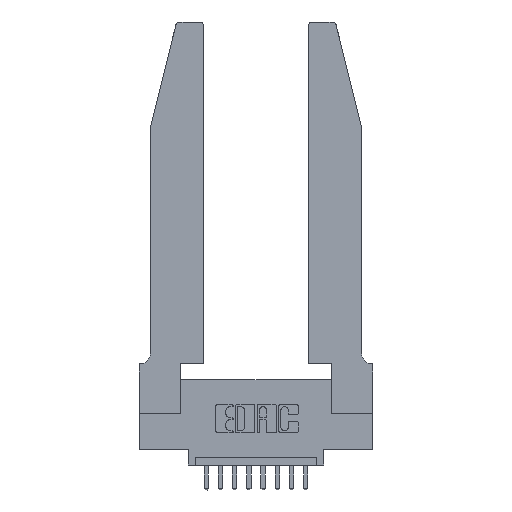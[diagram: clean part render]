
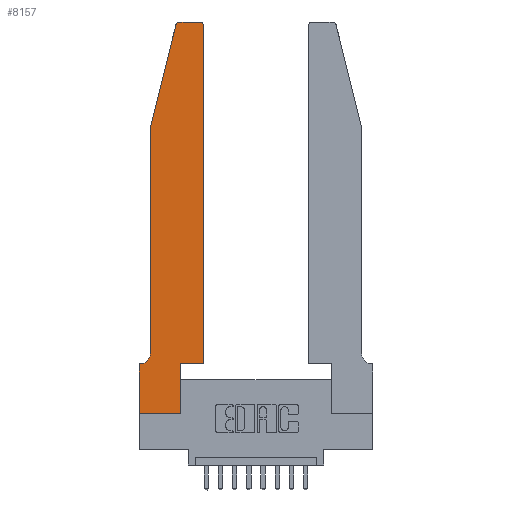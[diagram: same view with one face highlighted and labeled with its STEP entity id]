
A CAD part, top view. The second image highlights one B-rep face of the part: STEP entity #8157.
In plain terms, the highlighted planar face has unit normal (0, 0, 1).
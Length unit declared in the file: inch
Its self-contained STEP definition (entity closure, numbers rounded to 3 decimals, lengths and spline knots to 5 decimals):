
#4 = VECTOR ( 'NONE', #285, 39.37008 ) ;
#128 = EDGE_CURVE ( 'NONE', #5290, #318, #14136, .T. ) ;
#135 = CIRCLE ( 'NONE', #1114, 0.07 ) ;
#285 = DIRECTION ( 'NONE',  ( -1., 0., 0. ) ) ;
#318 = VERTEX_POINT ( 'NONE', #3411 ) ;
#564 = ORIENTED_EDGE ( 'NONE', *, *, #2130, .T. ) ;
#979 = VERTEX_POINT ( 'NONE', #3110 ) ;
#990 = DIRECTION ( 'NONE',  ( -0.239, -0.971, 0. ) ) ;
#1001 = AXIS2_PLACEMENT_3D ( 'NONE', #14861, #8774, #15068 ) ;
#1114 = AXIS2_PLACEMENT_3D ( 'NONE', #7270, #13454, #8474 ) ;
#1178 = DIRECTION ( 'NONE',  ( 1., 0., 0. ) ) ;
#1320 = DIRECTION ( 'NONE',  ( 0., -1., 0. ) ) ;
#1664 = CIRCLE ( 'NONE', #12497, 0.03 ) ;
#1901 = CARTESIAN_POINT ( 'NONE',  ( 0., 0.35, 0.37 ) ) ;
#2130 = EDGE_CURVE ( 'NONE', #8132, #9506, #135, .T. ) ;
#2642 = VERTEX_POINT ( 'NONE', #6205 ) ;
#3025 = EDGE_CURVE ( 'NONE', #9506, #979, #5407, .T. ) ;
#3107 = LINE ( 'NONE', #11360, #7609 ) ;
#3110 = CARTESIAN_POINT ( 'NONE',  ( 0., 0.35, 0.37 ) ) ;
#3137 = DIRECTION ( 'NONE',  ( 0., 0., 1. ) ) ;
#3411 = CARTESIAN_POINT ( 'NONE',  ( 0.4205, 2.75, 0.37 ) ) ;
#3567 = CARTESIAN_POINT ( 'NONE',  ( 0.4505, 0.35, 0.37 ) ) ;
#4018 = LINE ( 'NONE', #10999, #4 ) ;
#4222 = CARTESIAN_POINT ( 'NONE',  ( 0.0755, 2., 0.37 ) ) ;
#4379 = ORIENTED_EDGE ( 'NONE', *, *, #10028, .T. ) ;
#4506 = ORIENTED_EDGE ( 'NONE', *, *, #12321, .T. ) ;
#4670 = CARTESIAN_POINT ( 'NONE',  ( 0.0055, 0.35, 0.37 ) ) ;
#4680 = EDGE_CURVE ( 'NONE', #4938, #5290, #9488, .T. ) ;
#4683 = LINE ( 'NONE', #13005, #7518 ) ;
#4880 = DIRECTION ( 'NONE',  ( 0., 1., 0. ) ) ;
#4938 = VERTEX_POINT ( 'NONE', #3567 ) ;
#4985 = ORIENTED_EDGE ( 'NONE', *, *, #8995, .T. ) ;
#5169 = VERTEX_POINT ( 'NONE', #12025 ) ;
#5290 = VERTEX_POINT ( 'NONE', #15595 ) ;
#5407 = LINE ( 'NONE', #6294, #13510 ) ;
#5661 = EDGE_CURVE ( 'NONE', #7290, #8132, #3107, .T. ) ;
#6205 = CARTESIAN_POINT ( 'NONE',  ( 0.284, 2.75, 0.37 ) ) ;
#6294 = CARTESIAN_POINT ( 'NONE',  ( 0.0755, 0.35, 0.37 ) ) ;
#6397 = VECTOR ( 'NONE', #15098, 39.37008 ) ;
#6415 = ORIENTED_EDGE ( 'NONE', *, *, #3025, .T. ) ;
#6517 = CARTESIAN_POINT ( 'NONE',  ( 0., 0., 0.37 ) ) ;
#6561 = DIRECTION ( 'NONE',  ( 0., 0., 1. ) ) ;
#6606 = EDGE_CURVE ( 'NONE', #979, #14079, #13800, .T. ) ;
#6662 = CARTESIAN_POINT ( 'NONE',  ( 0.284, 2.72, 0.37 ) ) ;
#7002 = ORIENTED_EDGE ( 'NONE', *, *, #128, .T. ) ;
#7270 = CARTESIAN_POINT ( 'NONE',  ( 0.0055, 0.42, 0.37 ) ) ;
#7290 = VERTEX_POINT ( 'NONE', #4222 ) ;
#7411 = VECTOR ( 'NONE', #1178, 39.37008 ) ;
#7518 = VECTOR ( 'NONE', #990, 39.37008 ) ;
#7577 = VECTOR ( 'NONE', #1320, 39.37008 ) ;
#7609 = VECTOR ( 'NONE', #9970, 39.37008 ) ;
#7631 = VERTEX_POINT ( 'NONE', #7920 ) ;
#7920 = CARTESIAN_POINT ( 'NONE',  ( 0.25487, 2.72718, 0.37 ) ) ;
#8132 = VERTEX_POINT ( 'NONE', #10089 ) ;
#8149 = ORIENTED_EDGE ( 'NONE', *, *, #14007, .T. ) ;
#8157 = ADVANCED_FACE ( 'NONE', ( #12020 ), #13825, .T. ) ;
#8233 = EDGE_CURVE ( 'NONE', #11863, #5169, #8821, .T. ) ;
#8285 = ORIENTED_EDGE ( 'NONE', *, *, #6606, .T. ) ;
#8392 = CARTESIAN_POINT ( 'NONE',  ( 0.4505, 0.35, 0.37 ) ) ;
#8474 = DIRECTION ( 'NONE',  ( -1., 0., 0. ) ) ;
#8525 = CARTESIAN_POINT ( 'NONE',  ( 0.4505, 0.35, 0.37 ) ) ;
#8774 = DIRECTION ( 'NONE',  ( 0., 0., 1. ) ) ;
#8821 = LINE ( 'NONE', #15002, #6397 ) ;
#8922 = ORIENTED_EDGE ( 'NONE', *, *, #9254, .T. ) ;
#8995 = EDGE_CURVE ( 'NONE', #2642, #7631, #1664, .T. ) ;
#9141 = AXIS2_PLACEMENT_3D ( 'NONE', #1901, #3137, #13769 ) ;
#9254 = EDGE_CURVE ( 'NONE', #7631, #7290, #4683, .T. ) ;
#9488 = LINE ( 'NONE', #8392, #12331 ) ;
#9506 = VERTEX_POINT ( 'NONE', #4670 ) ;
#9832 = CARTESIAN_POINT ( 'NONE',  ( 0., 0., 0.37 ) ) ;
#9970 = DIRECTION ( 'NONE',  ( 0., -1., 0. ) ) ;
#9994 = DIRECTION ( 'NONE',  ( -1., 0., 0. ) ) ;
#10028 = EDGE_CURVE ( 'NONE', #5169, #4938, #12949, .T. ) ;
#10089 = CARTESIAN_POINT ( 'NONE',  ( 0.0755, 0.42, 0.37 ) ) ;
#10721 = DIRECTION ( 'NONE',  ( 1., 0., 0. ) ) ;
#10999 = CARTESIAN_POINT ( 'NONE',  ( 0.2605, 2.75, 0.37 ) ) ;
#11360 = CARTESIAN_POINT ( 'NONE',  ( 0.0755, 2., 0.37 ) ) ;
#11863 = VERTEX_POINT ( 'NONE', #13721 ) ;
#12020 = FACE_OUTER_BOUND ( 'NONE', #15440, .T. ) ;
#12025 = CARTESIAN_POINT ( 'NONE',  ( 0.2865, 0.35, 0.37 ) ) ;
#12254 = ORIENTED_EDGE ( 'NONE', *, *, #8233, .T. ) ;
#12321 = EDGE_CURVE ( 'NONE', #14079, #11863, #13655, .T. ) ;
#12331 = VECTOR ( 'NONE', #4880, 39.37008 ) ;
#12497 = AXIS2_PLACEMENT_3D ( 'NONE', #6662, #6561, #13667 ) ;
#12877 = ORIENTED_EDGE ( 'NONE', *, *, #4680, .T. ) ;
#12949 = LINE ( 'NONE', #8525, #13729 ) ;
#13005 = CARTESIAN_POINT ( 'NONE',  ( 0.0755, 2., 0.37 ) ) ;
#13454 = DIRECTION ( 'NONE',  ( 0., 0., -1. ) ) ;
#13504 = ORIENTED_EDGE ( 'NONE', *, *, #5661, .T. ) ;
#13510 = VECTOR ( 'NONE', #9994, 39.37008 ) ;
#13655 = LINE ( 'NONE', #15551, #7411 ) ;
#13667 = DIRECTION ( 'NONE',  ( 1., 0., 0. ) ) ;
#13721 = CARTESIAN_POINT ( 'NONE',  ( 0.2865, 0., 0.37 ) ) ;
#13729 = VECTOR ( 'NONE', #10721, 39.37008 ) ;
#13769 = DIRECTION ( 'NONE',  ( 1., 0., 0. ) ) ;
#13800 = LINE ( 'NONE', #9832, #7577 ) ;
#13825 = PLANE ( 'NONE',  #9141 ) ;
#14007 = EDGE_CURVE ( 'NONE', #318, #2642, #4018, .T. ) ;
#14079 = VERTEX_POINT ( 'NONE', #6517 ) ;
#14136 = CIRCLE ( 'NONE', #1001, 0.03 ) ;
#14861 = CARTESIAN_POINT ( 'NONE',  ( 0.4205, 2.72, 0.37 ) ) ;
#15002 = CARTESIAN_POINT ( 'NONE',  ( 0.2865, 0.35, 0.37 ) ) ;
#15068 = DIRECTION ( 'NONE',  ( 1., 0., 0. ) ) ;
#15098 = DIRECTION ( 'NONE',  ( 0., 1., 0. ) ) ;
#15440 = EDGE_LOOP ( 'NONE', ( #8149, #4985, #8922, #13504, #564, #6415, #8285, #4506, #12254, #4379, #12877, #7002 ) ) ;
#15551 = CARTESIAN_POINT ( 'NONE',  ( 0., 0., 0.37 ) ) ;
#15595 = CARTESIAN_POINT ( 'NONE',  ( 0.4505, 2.72, 0.37 ) ) ;
